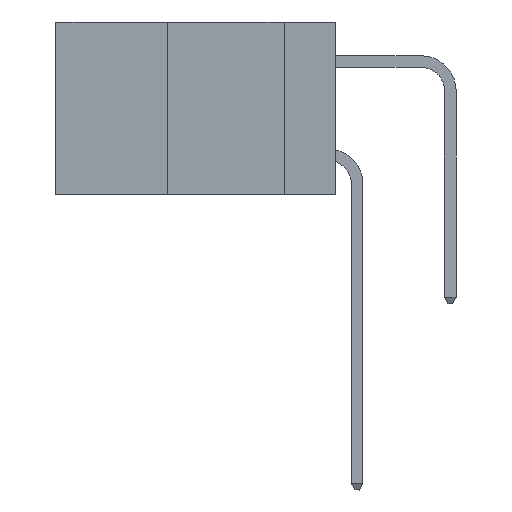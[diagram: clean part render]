
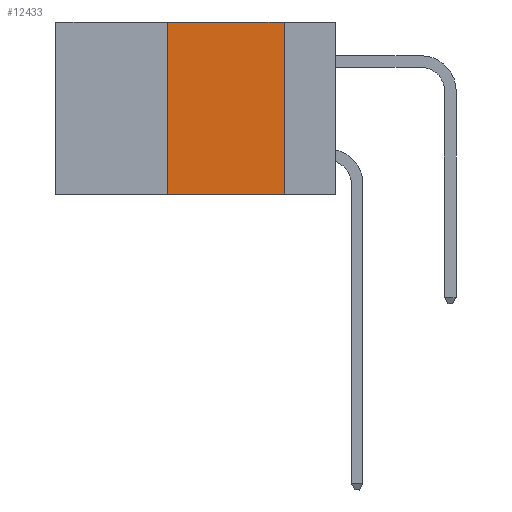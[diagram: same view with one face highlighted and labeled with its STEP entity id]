
A CAD part, left-side view. The second image highlights one B-rep face of the part: STEP entity #12433.
In plain terms, the highlighted planar face has unit normal (-1, 0, 0).
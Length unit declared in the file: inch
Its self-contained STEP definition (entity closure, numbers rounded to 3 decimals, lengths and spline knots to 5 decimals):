
#935 = CARTESIAN_POINT ( 'NONE',  ( 0., 0.6, 0. ) ) ;
#1056 = EDGE_CURVE ( 'NONE', #23589, #3402, #3091, .T. ) ;
#2113 = CARTESIAN_POINT ( 'NONE',  ( 0., 0.11, 0. ) ) ;
#3091 = LINE ( 'NONE', #43084, #19785 ) ;
#3402 = VERTEX_POINT ( 'NONE', #12705 ) ;
#4154 = EDGE_LOOP ( 'NONE', ( #35737, #22802, #12397, #34381 ) ) ;
#7887 = CARTESIAN_POINT ( 'NONE',  ( 0., 0.6, -0.37 ) ) ;
#8775 = DIRECTION ( 'NONE',  ( 0., 0., -1. ) ) ;
#10928 = CARTESIAN_POINT ( 'NONE',  ( 0., 0.11, -0.37 ) ) ;
#12064 = CARTESIAN_POINT ( 'NONE',  ( 0., 0.6, 0. ) ) ;
#12397 = ORIENTED_EDGE ( 'NONE', *, *, #1056, .F. ) ;
#12433 = ADVANCED_FACE ( 'NONE', ( #35259 ), #24885, .F. ) ;
#12705 = CARTESIAN_POINT ( 'NONE',  ( 0., 0.36, 0. ) ) ;
#13010 = AXIS2_PLACEMENT_3D ( 'NONE', #12064, #31963, #24652 ) ;
#13744 = EDGE_CURVE ( 'NONE', #15107, #35528, #25103, .T. ) ;
#15107 = VERTEX_POINT ( 'NONE', #2113 ) ;
#16260 = VECTOR ( 'NONE', #8775, 39.37008 ) ;
#16521 = VECTOR ( 'NONE', #28310, 39.37008 ) ;
#19465 = DIRECTION ( 'NONE',  ( 0., 0., 1. ) ) ;
#19785 = VECTOR ( 'NONE', #19465, 39.37008 ) ;
#20682 = CARTESIAN_POINT ( 'NONE',  ( 0., 0.36, -0.37 ) ) ;
#22802 = ORIENTED_EDGE ( 'NONE', *, *, #29590, .F. ) ;
#23589 = VERTEX_POINT ( 'NONE', #20682 ) ;
#24638 = DIRECTION ( 'NONE',  ( 0., -1., 0. ) ) ;
#24652 = DIRECTION ( 'NONE',  ( 0., 0., -1. ) ) ;
#24885 = PLANE ( 'NONE',  #13010 ) ;
#24970 = EDGE_CURVE ( 'NONE', #23589, #35528, #35246, .T. ) ;
#25103 = LINE ( 'NONE', #34845, #16260 ) ;
#28310 = DIRECTION ( 'NONE',  ( 0., -1., 0. ) ) ;
#29590 = EDGE_CURVE ( 'NONE', #3402, #15107, #31430, .T. ) ;
#31430 = LINE ( 'NONE', #935, #16521 ) ;
#31963 = DIRECTION ( 'NONE',  ( 1., 0., 0. ) ) ;
#34381 = ORIENTED_EDGE ( 'NONE', *, *, #24970, .T. ) ;
#34845 = CARTESIAN_POINT ( 'NONE',  ( 0., 0.11, 0. ) ) ;
#35246 = LINE ( 'NONE', #7887, #42455 ) ;
#35259 = FACE_OUTER_BOUND ( 'NONE', #4154, .T. ) ;
#35528 = VERTEX_POINT ( 'NONE', #10928 ) ;
#35737 = ORIENTED_EDGE ( 'NONE', *, *, #13744, .F. ) ;
#42455 = VECTOR ( 'NONE', #24638, 39.37008 ) ;
#43084 = CARTESIAN_POINT ( 'NONE',  ( 0., 0.36, 0. ) ) ;
